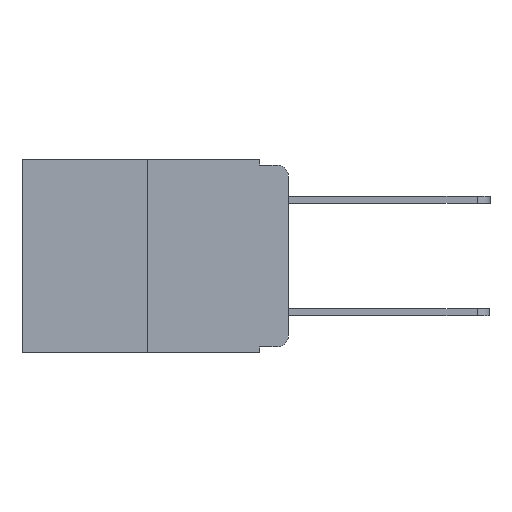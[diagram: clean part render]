
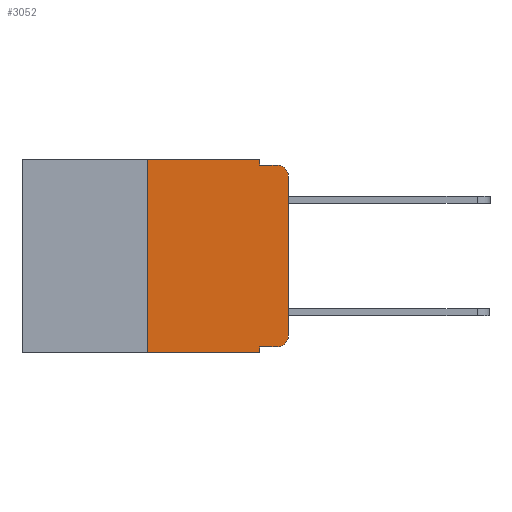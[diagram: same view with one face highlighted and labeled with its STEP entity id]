
A CAD part, left-side view. The second image highlights one B-rep face of the part: STEP entity #3052.
In plain terms, the highlighted planar face has unit normal (-1, 0, 0).
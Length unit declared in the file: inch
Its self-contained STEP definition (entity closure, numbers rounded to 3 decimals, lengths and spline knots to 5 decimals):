
#103 = AXIS2_PLACEMENT_3D ( 'NONE', #13830, #10020, #9958 ) ;
#132 = DIRECTION ( 'NONE',  ( 0., 0., 1. ) ) ;
#428 = VECTOR ( 'NONE', #16061, 39.37008 ) ;
#621 = EDGE_CURVE ( 'NONE', #4955, #10095, #13046, .T. ) ;
#856 = ORIENTED_EDGE ( 'NONE', *, *, #1238, .T. ) ;
#1135 = ORIENTED_EDGE ( 'NONE', *, *, #1538, .F. ) ;
#1238 = EDGE_CURVE ( 'NONE', #8073, #4582, #14575, .T. ) ;
#1477 = EDGE_CURVE ( 'NONE', #1945, #7947, #4815, .T. ) ;
#1482 = EDGE_CURVE ( 'NONE', #7947, #12194, #8789, .T. ) ;
#1510 = EDGE_CURVE ( 'NONE', #10271, #12194, #15687, .T. ) ;
#1511 = EDGE_CURVE ( 'NONE', #10095, #10271, #14925, .T. ) ;
#1538 = EDGE_CURVE ( 'NONE', #8073, #4955, #11162, .T. ) ;
#1539 = EDGE_CURVE ( 'NONE', #13154, #4582, #7409, .T. ) ;
#1540 = EDGE_CURVE ( 'NONE', #13154, #2914, #14175, .T. ) ;
#1541 = CARTESIAN_POINT ( 'NONE',  ( 0., 0.25, 0. ) ) ;
#1574 = EDGE_CURVE ( 'NONE', #2914, #1945, #10743, .T. ) ;
#1858 = ORIENTED_EDGE ( 'NONE', *, *, #621, .F. ) ;
#1945 = VERTEX_POINT ( 'NONE', #14672 ) ;
#2073 = CARTESIAN_POINT ( 'NONE',  ( 0., 0.051, 0. ) ) ;
#2302 = AXIS2_PLACEMENT_3D ( 'NONE', #14754, #14750, #14739 ) ;
#2524 = CARTESIAN_POINT ( 'NONE',  ( 0., 0.051, -0.333 ) ) ;
#2676 = CARTESIAN_POINT ( 'NONE',  ( 0., 0.02, -0.333 ) ) ;
#2771 = PLANE ( 'NONE',  #16194 ) ;
#2914 = VERTEX_POINT ( 'NONE', #2676 ) ;
#3052 = ADVANCED_FACE ( 'NONE', ( #7149 ), #2771, .F. ) ;
#3264 = VECTOR ( 'NONE', #17135, 39.37008 ) ;
#4022 = ORIENTED_EDGE ( 'NONE', *, *, #1482, .T. ) ;
#4057 = DIRECTION ( 'NONE',  ( 0., 0., -1. ) ) ;
#4161 = CARTESIAN_POINT ( 'NONE',  ( 0., 0.473, 0. ) ) ;
#4299 = CARTESIAN_POINT ( 'NONE',  ( 0., 0.25, -0.343 ) ) ;
#4582 = VERTEX_POINT ( 'NONE', #6645 ) ;
#4815 = LINE ( 'NONE', #10338, #428 ) ;
#4955 = VERTEX_POINT ( 'NONE', #4967 ) ;
#4967 = CARTESIAN_POINT ( 'NONE',  ( 0., 0.25, 0. ) ) ;
#5090 = CARTESIAN_POINT ( 'NONE',  ( 0., 0.473, 0. ) ) ;
#5110 = VECTOR ( 'NONE', #5206, 39.37008 ) ;
#5206 = DIRECTION ( 'NONE',  ( 0., -1., 0. ) ) ;
#5394 = DIRECTION ( 'NONE',  ( 0., 0., -1. ) ) ;
#5421 = DIRECTION ( 'NONE',  ( 1., 0., 0. ) ) ;
#5670 = ORIENTED_EDGE ( 'NONE', *, *, #1477, .T. ) ;
#5733 = ORIENTED_EDGE ( 'NONE', *, *, #1539, .F. ) ;
#6645 = CARTESIAN_POINT ( 'NONE',  ( 0., 0.051, -0.343 ) ) ;
#6929 = VECTOR ( 'NONE', #14274, 39.37008 ) ;
#7149 = FACE_OUTER_BOUND ( 'NONE', #17267, .T. ) ;
#7256 = ORIENTED_EDGE ( 'NONE', *, *, #1511, .F. ) ;
#7409 = LINE ( 'NONE', #2073, #3264 ) ;
#7562 = ORIENTED_EDGE ( 'NONE', *, *, #1510, .F. ) ;
#7947 = VERTEX_POINT ( 'NONE', #8522 ) ;
#8006 = CARTESIAN_POINT ( 'NONE',  ( 0., 0.02, -0.01 ) ) ;
#8073 = VERTEX_POINT ( 'NONE', #4299 ) ;
#8522 = CARTESIAN_POINT ( 'NONE',  ( 0., 0., -0.03 ) ) ;
#8789 = CIRCLE ( 'NONE', #103, 0.02 ) ;
#9204 = CARTESIAN_POINT ( 'NONE',  ( 0., 0.051, -0.01 ) ) ;
#9886 = ORIENTED_EDGE ( 'NONE', *, *, #1574, .T. ) ;
#9958 = DIRECTION ( 'NONE',  ( 0., 0., -1. ) ) ;
#10020 = DIRECTION ( 'NONE',  ( -1., 0., 0. ) ) ;
#10095 = VERTEX_POINT ( 'NONE', #17385 ) ;
#10271 = VERTEX_POINT ( 'NONE', #11454 ) ;
#10338 = CARTESIAN_POINT ( 'NONE',  ( 0., 0., 0. ) ) ;
#10743 = CIRCLE ( 'NONE', #2302, 0.02 ) ;
#11162 = LINE ( 'NONE', #1541, #17403 ) ;
#11454 = CARTESIAN_POINT ( 'NONE',  ( 0., 0.051, -0.01 ) ) ;
#11567 = VECTOR ( 'NONE', #15486, 39.37008 ) ;
#12194 = VERTEX_POINT ( 'NONE', #8006 ) ;
#13046 = LINE ( 'NONE', #5090, #5110 ) ;
#13154 = VERTEX_POINT ( 'NONE', #2524 ) ;
#13830 = CARTESIAN_POINT ( 'NONE',  ( 0., 0.02, -0.03 ) ) ;
#14175 = LINE ( 'NONE', #16869, #6929 ) ;
#14274 = DIRECTION ( 'NONE',  ( 0., -1., 0. ) ) ;
#14575 = LINE ( 'NONE', #15016, #17045 ) ;
#14672 = CARTESIAN_POINT ( 'NONE',  ( 0., 0., -0.313 ) ) ;
#14739 = DIRECTION ( 'NONE',  ( 0., 0., -1. ) ) ;
#14750 = DIRECTION ( 'NONE',  ( -1., 0., 0. ) ) ;
#14754 = CARTESIAN_POINT ( 'NONE',  ( 0., 0.02, -0.313 ) ) ;
#14925 = LINE ( 'NONE', #15452, #15287 ) ;
#15016 = CARTESIAN_POINT ( 'NONE',  ( 0., 0.473, -0.343 ) ) ;
#15287 = VECTOR ( 'NONE', #4057, 39.37008 ) ;
#15452 = CARTESIAN_POINT ( 'NONE',  ( 0., 0.051, 0. ) ) ;
#15486 = DIRECTION ( 'NONE',  ( 0., -1., 0. ) ) ;
#15687 = LINE ( 'NONE', #9204, #11567 ) ;
#15742 = DIRECTION ( 'NONE',  ( 0., -1., 0. ) ) ;
#16061 = DIRECTION ( 'NONE',  ( 0., 0., 1. ) ) ;
#16194 = AXIS2_PLACEMENT_3D ( 'NONE', #4161, #5421, #5394 ) ;
#16869 = CARTESIAN_POINT ( 'NONE',  ( 0., 0.051, -0.333 ) ) ;
#17045 = VECTOR ( 'NONE', #15742, 39.37008 ) ;
#17135 = DIRECTION ( 'NONE',  ( 0., 0., -1. ) ) ;
#17203 = ORIENTED_EDGE ( 'NONE', *, *, #1540, .T. ) ;
#17267 = EDGE_LOOP ( 'NONE', ( #5670, #4022, #7562, #7256, #1858, #1135, #856, #5733, #17203, #9886 ) ) ;
#17385 = CARTESIAN_POINT ( 'NONE',  ( 0., 0.051, 0. ) ) ;
#17403 = VECTOR ( 'NONE', #132, 39.37008 ) ;
